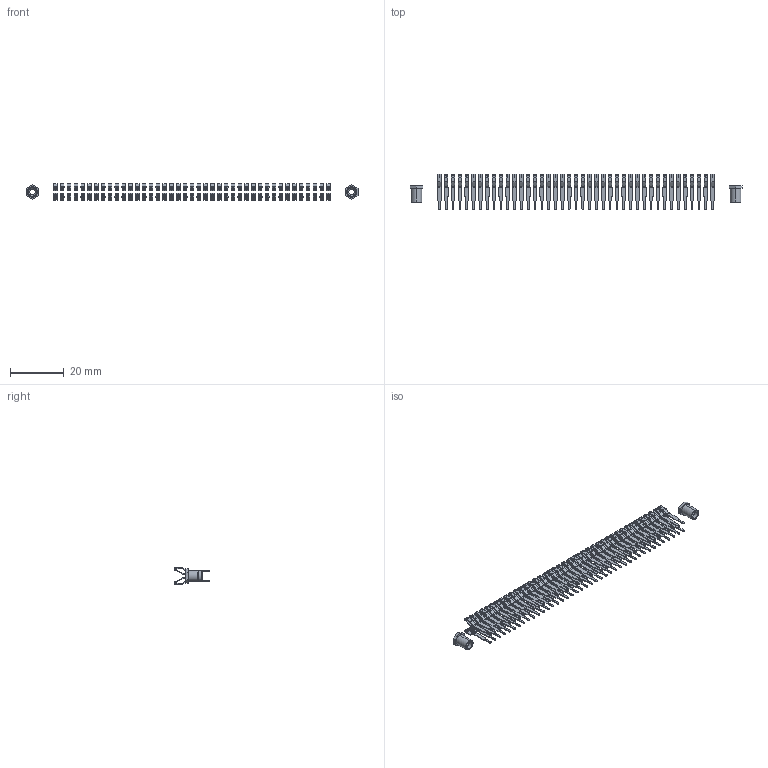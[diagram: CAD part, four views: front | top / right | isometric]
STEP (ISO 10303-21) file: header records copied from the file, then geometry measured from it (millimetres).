
FILE_DESCRIPTION (( 'STEP AP203' ), '1' );
FILE_NAME ('341-082-524-208.STEP', '2018-08-07T22:14:46', ( '' ), ( '' ), 'SwSTEP 2.0', 'SolidWorks 2016', '' );
FILE_SCHEMA (( 'CONFIG_CONTROL_DESIGN' ));
Length unit declared in the file: inch
Products named in the file (4): 341 Part_.156 (3.96) Dia Mounting Holes; 341-292-001_341-292-124; 345-250-001_345-250-003-102; 341-082-524-208
Assembly tree (85 placements, depth 2):
  341-082-524-208
    341 Part_.156 (3.96) Dia Mounting Holes
    341-292-001_341-292-124  x82
    345-250-001_345-250-003-102  x2
Bounding box: 123.49 x 13.13 x 6.25 mm (x, y, z)
Volume: 678.5 mm3; surface area: 5261.9 mm2
Topology: 84 solids, 84 shells, 4146 faces, 12072 edges, 7932 vertices
Faces by surface type: plane 2396, cylinder 1734, cone 12, torus 4
Entity records: 50937 total; most frequent: CARTESIAN_POINT 8450, ORIENTED_EDGE 8390, DIRECTION 8211, EDGE_CURVE 4195, VECTOR 3385, LINE 3385, VERTEX_POINT 2652, AXIS2_PLACEMENT_3D 2413
